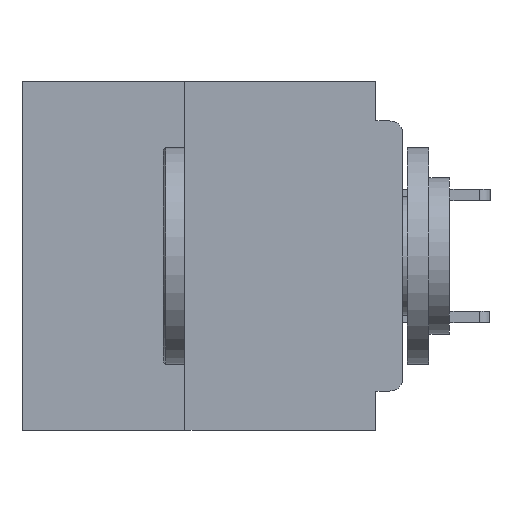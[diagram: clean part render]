
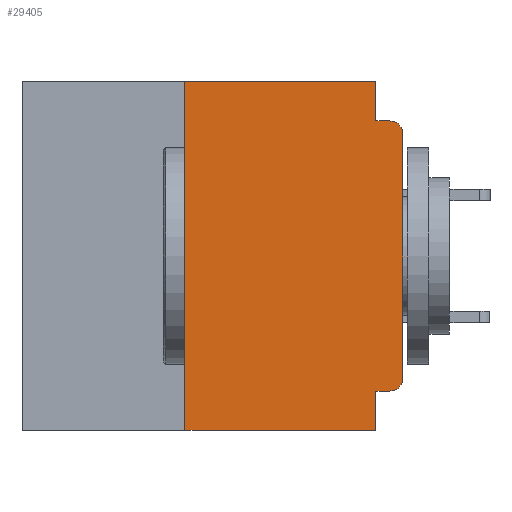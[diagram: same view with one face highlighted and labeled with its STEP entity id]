
A CAD part, left-side view. The second image highlights one B-rep face of the part: STEP entity #29405.
In plain terms, the highlighted planar face has unit normal (-1, 0, 0).
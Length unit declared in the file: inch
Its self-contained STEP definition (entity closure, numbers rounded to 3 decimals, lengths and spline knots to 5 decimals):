
#667 = CIRCLE ( 'NONE', #25878, 0.015 ) ;
#1061 = CARTESIAN_POINT ( 'NONE',  ( 0., 0.031, -0.4 ) ) ;
#1452 = CARTESIAN_POINT ( 'NONE',  ( 0., 0.031, 0. ) ) ;
#1653 = CARTESIAN_POINT ( 'NONE',  ( 0., 0.25, 0. ) ) ;
#2982 = ORIENTED_EDGE ( 'NONE', *, *, #13422, .T. ) ;
#3850 = PLANE ( 'NONE',  #44658 ) ;
#4223 = VECTOR ( 'NONE', #41922, 39.37008 ) ;
#5117 = DIRECTION ( 'NONE',  ( 0., 0., -1. ) ) ;
#5463 = CARTESIAN_POINT ( 'NONE',  ( 0., 0.015, -0.06 ) ) ;
#7448 = EDGE_CURVE ( 'NONE', #27324, #15359, #11461, .T. ) ;
#7490 = ORIENTED_EDGE ( 'NONE', *, *, #17487, .F. ) ;
#8334 = EDGE_CURVE ( 'NONE', #27324, #14148, #10285, .T. ) ;
#8435 = VERTEX_POINT ( 'NONE', #37519 ) ;
#8777 = EDGE_CURVE ( 'NONE', #42854, #32513, #667, .T. ) ;
#9010 = EDGE_CURVE ( 'NONE', #8435, #36273, #27224, .T. ) ;
#9074 = DIRECTION ( 'NONE',  ( 0., 0., -1. ) ) ;
#9484 = CARTESIAN_POINT ( 'NONE',  ( 0., 0.031, -0.4 ) ) ;
#10285 = LINE ( 'NONE', #36919, #37036 ) ;
#10321 = ORIENTED_EDGE ( 'NONE', *, *, #8777, .T. ) ;
#11002 = VECTOR ( 'NONE', #5117, 39.37008 ) ;
#11035 = DIRECTION ( 'NONE',  ( 0., 0., -1. ) ) ;
#11461 = LINE ( 'NONE', #28279, #19671 ) ;
#11900 = DIRECTION ( 'NONE',  ( 0., 0., -1. ) ) ;
#13422 = EDGE_CURVE ( 'NONE', #15008, #36273, #32713, .T. ) ;
#14148 = VERTEX_POINT ( 'NONE', #9484 ) ;
#14260 = CARTESIAN_POINT ( 'NONE',  ( 0., 0.25, -0.4 ) ) ;
#15008 = VERTEX_POINT ( 'NONE', #24459 ) ;
#15197 = EDGE_LOOP ( 'NONE', ( #45129, #2982, #40291, #7490, #35449, #29501, #31674, #15232, #18525, #10321 ) ) ;
#15232 = ORIENTED_EDGE ( 'NONE', *, *, #34978, .F. ) ;
#15359 = VERTEX_POINT ( 'NONE', #1653 ) ;
#17024 = FACE_OUTER_BOUND ( 'NONE', #15197, .T. ) ;
#17487 = EDGE_CURVE ( 'NONE', #27177, #8435, #38846, .T. ) ;
#17575 = CARTESIAN_POINT ( 'NONE',  ( 0., 0., 0. ) ) ;
#17870 = VECTOR ( 'NONE', #19792, 39.37008 ) ;
#18401 = CARTESIAN_POINT ( 'NONE',  ( 0., 0.437, 0. ) ) ;
#18525 = ORIENTED_EDGE ( 'NONE', *, *, #37462, .F. ) ;
#18583 = DIRECTION ( 'NONE',  ( -1., 0., 0. ) ) ;
#19438 = LINE ( 'NONE', #37140, #28780 ) ;
#19671 = VECTOR ( 'NONE', #42016, 39.37008 ) ;
#19792 = DIRECTION ( 'NONE',  ( 0., -1., 0. ) ) ;
#20789 = VECTOR ( 'NONE', #35667, 39.37008 ) ;
#21811 = EDGE_CURVE ( 'NONE', #32513, #15008, #23006, .T. ) ;
#23006 = LINE ( 'NONE', #17575, #4223 ) ;
#23960 = CARTESIAN_POINT ( 'NONE',  ( 0., 0.031, 0. ) ) ;
#24459 = CARTESIAN_POINT ( 'NONE',  ( 0., 0., -0.06 ) ) ;
#24657 = CARTESIAN_POINT ( 'NONE',  ( 0., 0.031, -0.355 ) ) ;
#25878 = AXIS2_PLACEMENT_3D ( 'NONE', #39443, #18583, #42930 ) ;
#27177 = VERTEX_POINT ( 'NONE', #23960 ) ;
#27224 = LINE ( 'NONE', #30229, #17870 ) ;
#27324 = VERTEX_POINT ( 'NONE', #14260 ) ;
#28279 = CARTESIAN_POINT ( 'NONE',  ( 0., 0.25, -0.4 ) ) ;
#28780 = VECTOR ( 'NONE', #40624, 39.37008 ) ;
#29405 = ADVANCED_FACE ( 'NONE', ( #17024 ), #3850, .F. ) ;
#29501 = ORIENTED_EDGE ( 'NONE', *, *, #7448, .F. ) ;
#30103 = DIRECTION ( 'NONE',  ( -1., 0., 0. ) ) ;
#30151 = CARTESIAN_POINT ( 'NONE',  ( 0., 0., -0.34 ) ) ;
#30229 = CARTESIAN_POINT ( 'NONE',  ( 0., 0., -0.045 ) ) ;
#31674 = ORIENTED_EDGE ( 'NONE', *, *, #8334, .T. ) ;
#32011 = DIRECTION ( 'NONE',  ( 1., 0., 0. ) ) ;
#32513 = VERTEX_POINT ( 'NONE', #30151 ) ;
#32713 = CIRCLE ( 'NONE', #36202, 0.015 ) ;
#33242 = CARTESIAN_POINT ( 'NONE',  ( 0., 0.015, -0.355 ) ) ;
#34744 = VECTOR ( 'NONE', #11900, 39.37008 ) ;
#34978 = EDGE_CURVE ( 'NONE', #41187, #14148, #43910, .T. ) ;
#35449 = ORIENTED_EDGE ( 'NONE', *, *, #40747, .F. ) ;
#35667 = DIRECTION ( 'NONE',  ( 0., -1., 0. ) ) ;
#36202 = AXIS2_PLACEMENT_3D ( 'NONE', #5463, #30103, #9074 ) ;
#36273 = VERTEX_POINT ( 'NONE', #36528 ) ;
#36528 = CARTESIAN_POINT ( 'NONE',  ( 0., 0.015, -0.045 ) ) ;
#36919 = CARTESIAN_POINT ( 'NONE',  ( 0., 0.437, -0.4 ) ) ;
#37036 = VECTOR ( 'NONE', #40393, 39.37008 ) ;
#37140 = CARTESIAN_POINT ( 'NONE',  ( 0., 0., -0.355 ) ) ;
#37462 = EDGE_CURVE ( 'NONE', #42854, #41187, #19438, .T. ) ;
#37519 = CARTESIAN_POINT ( 'NONE',  ( 0., 0.031, -0.045 ) ) ;
#38846 = LINE ( 'NONE', #1452, #11002 ) ;
#39443 = CARTESIAN_POINT ( 'NONE',  ( 0., 0.015, -0.34 ) ) ;
#40291 = ORIENTED_EDGE ( 'NONE', *, *, #9010, .F. ) ;
#40393 = DIRECTION ( 'NONE',  ( 0., -1., 0. ) ) ;
#40624 = DIRECTION ( 'NONE',  ( 0., 1., 0. ) ) ;
#40747 = EDGE_CURVE ( 'NONE', #15359, #27177, #44704, .T. ) ;
#41187 = VERTEX_POINT ( 'NONE', #24657 ) ;
#41922 = DIRECTION ( 'NONE',  ( 0., 0., 1. ) ) ;
#42016 = DIRECTION ( 'NONE',  ( 0., 0., 1. ) ) ;
#42268 = CARTESIAN_POINT ( 'NONE',  ( 0., 0.437, 0. ) ) ;
#42854 = VERTEX_POINT ( 'NONE', #33242 ) ;
#42930 = DIRECTION ( 'NONE',  ( 0., 0., -1. ) ) ;
#43910 = LINE ( 'NONE', #1061, #34744 ) ;
#44658 = AXIS2_PLACEMENT_3D ( 'NONE', #42268, #32011, #11035 ) ;
#44704 = LINE ( 'NONE', #18401, #20789 ) ;
#45129 = ORIENTED_EDGE ( 'NONE', *, *, #21811, .T. ) ;
